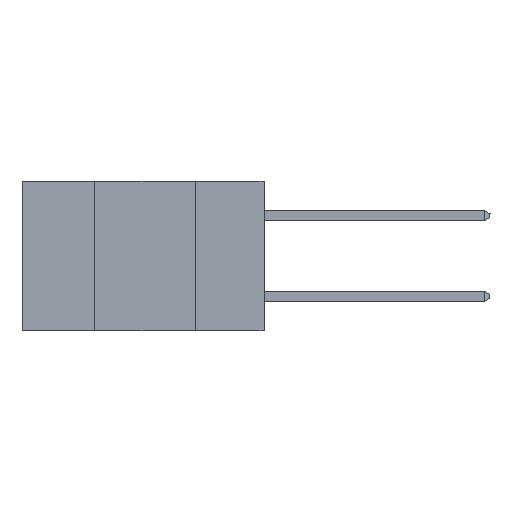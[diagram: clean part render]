
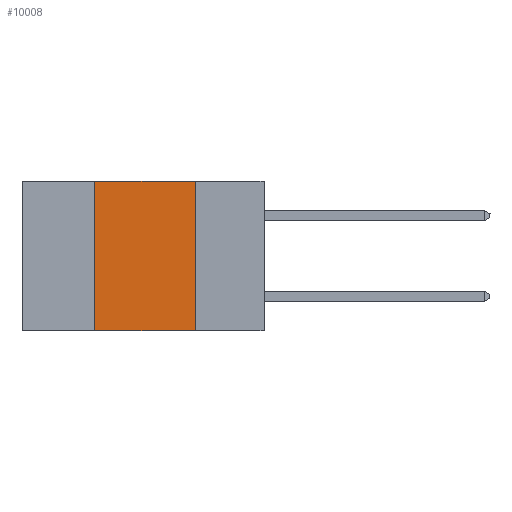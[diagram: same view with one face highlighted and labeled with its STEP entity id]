
A CAD part, left-side view. The second image highlights one B-rep face of the part: STEP entity #10008.
In plain terms, the highlighted planar face has unit normal (-1, 0, 0).
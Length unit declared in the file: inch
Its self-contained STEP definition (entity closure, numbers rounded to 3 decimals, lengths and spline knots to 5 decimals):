
#729 = LINE ( 'NONE', #7554, #24908 ) ;
#1223 = VECTOR ( 'NONE', #17343, 39.37008 ) ;
#1286 = AXIS2_PLACEMENT_3D ( 'NONE', #16362, #10616, #4818 ) ;
#1835 = EDGE_CURVE ( 'NONE', #6813, #2579, #2088, .T. ) ;
#1973 = LINE ( 'NONE', #10306, #1223 ) ;
#2088 = LINE ( 'NONE', #28579, #19437 ) ;
#2579 = VERTEX_POINT ( 'NONE', #26551 ) ;
#2793 = VERTEX_POINT ( 'NONE', #17629 ) ;
#4818 = DIRECTION ( 'NONE',  ( 0., 0., -1. ) ) ;
#6813 = VERTEX_POINT ( 'NONE', #14578 ) ;
#7554 = CARTESIAN_POINT ( 'NONE',  ( 0., 0.17, 0. ) ) ;
#7877 = CARTESIAN_POINT ( 'NONE',  ( 0., 0.17, -0.37 ) ) ;
#8372 = EDGE_LOOP ( 'NONE', ( #26590, #28708, #9550, #19473 ) ) ;
#9359 = DIRECTION ( 'NONE',  ( 0., 0., 1. ) ) ;
#9550 = ORIENTED_EDGE ( 'NONE', *, *, #1835, .F. ) ;
#10008 = ADVANCED_FACE ( 'NONE', ( #14378 ), #21315, .F. ) ;
#10306 = CARTESIAN_POINT ( 'NONE',  ( 0., 0.6, 0. ) ) ;
#10616 = DIRECTION ( 'NONE',  ( 1., 0., 0. ) ) ;
#13322 = VECTOR ( 'NONE', #16851, 39.37008 ) ;
#14378 = FACE_OUTER_BOUND ( 'NONE', #8372, .T. ) ;
#14483 = CARTESIAN_POINT ( 'NONE',  ( 0., 0.6, -0.37 ) ) ;
#14578 = CARTESIAN_POINT ( 'NONE',  ( 0., 0.42, -0.37 ) ) ;
#16362 = CARTESIAN_POINT ( 'NONE',  ( 0., 0.6, 0. ) ) ;
#16851 = DIRECTION ( 'NONE',  ( 0., -1., 0. ) ) ;
#17343 = DIRECTION ( 'NONE',  ( 0., -1., 0. ) ) ;
#17629 = CARTESIAN_POINT ( 'NONE',  ( 0., 0.17, 0. ) ) ;
#19437 = VECTOR ( 'NONE', #9359, 39.37008 ) ;
#19473 = ORIENTED_EDGE ( 'NONE', *, *, #24839, .T. ) ;
#21315 = PLANE ( 'NONE',  #1286 ) ;
#21595 = DIRECTION ( 'NONE',  ( 0., 0., -1. ) ) ;
#23040 = EDGE_CURVE ( 'NONE', #2579, #2793, #1973, .T. ) ;
#24839 = EDGE_CURVE ( 'NONE', #6813, #27079, #25625, .T. ) ;
#24874 = EDGE_CURVE ( 'NONE', #2793, #27079, #729, .T. ) ;
#24908 = VECTOR ( 'NONE', #21595, 39.37008 ) ;
#25625 = LINE ( 'NONE', #14483, #13322 ) ;
#26551 = CARTESIAN_POINT ( 'NONE',  ( 0., 0.42, 0. ) ) ;
#26590 = ORIENTED_EDGE ( 'NONE', *, *, #24874, .F. ) ;
#27079 = VERTEX_POINT ( 'NONE', #7877 ) ;
#28579 = CARTESIAN_POINT ( 'NONE',  ( 0., 0.42, 0. ) ) ;
#28708 = ORIENTED_EDGE ( 'NONE', *, *, #23040, .F. ) ;
